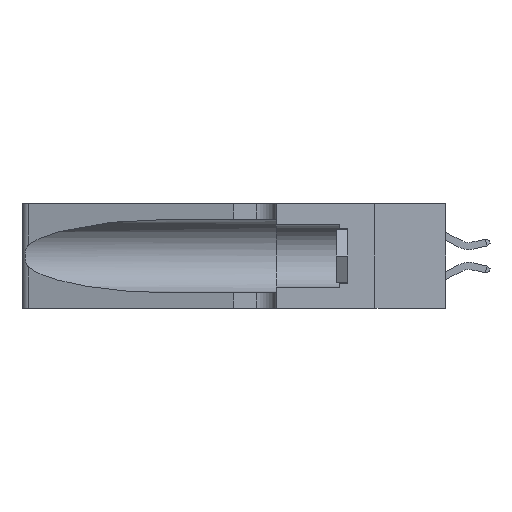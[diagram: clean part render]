
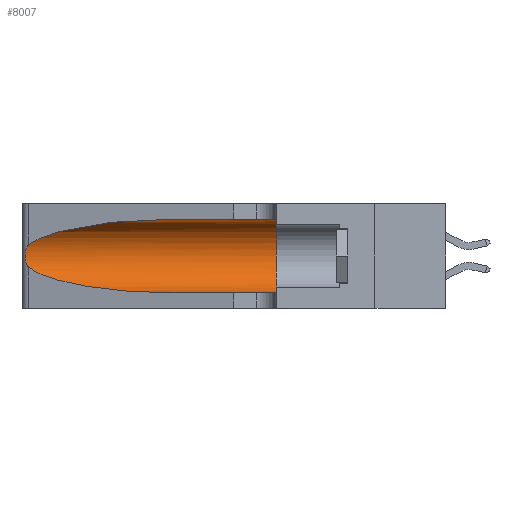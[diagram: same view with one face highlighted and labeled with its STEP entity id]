
A CAD part, left-side view. The second image highlights one B-rep face of the part: STEP entity #8007.
In plain terms, the highlighted cylindrical face has radius 3.308 mm (diameter 6.617 mm), a partial arc.
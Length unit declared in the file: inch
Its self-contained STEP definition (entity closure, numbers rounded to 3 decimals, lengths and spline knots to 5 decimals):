
#169 = VERTEX_POINT ( 'NONE', #20719 ) ;
#1342 = DIRECTION ( 'NONE',  ( 0., -1., 0. ) ) ;
#2211 = CARTESIAN_POINT ( 'NONE',  ( 0.25639, 1.23186, 0.15144 ) ) ;
#2343 = ORIENTED_EDGE ( 'NONE', *, *, #20347, .F. ) ;
#2468 = ORIENTED_EDGE ( 'NONE', *, *, #5573, .T. ) ;
#2977 = CARTESIAN_POINT ( 'NONE',  ( 0.1305, 0.35, 0.185 ) ) ;
#4000 = CARTESIAN_POINT ( 'NONE',  ( 0.1305, 1.61858, 0.31525 ) ) ;
#4860 = CARTESIAN_POINT ( 'NONE',  ( 0.25487, 1.22718, 0.14631 ) ) ;
#5573 = EDGE_CURVE ( 'NONE', #169, #20255, #29001, .T. ) ;
#5644 = CYLINDRICAL_SURFACE ( 'NONE', #11608, 0.13025 ) ;
#5645 = DIRECTION ( 'NONE',  ( 0., 0., 1. ) ) ;
#7001 = CARTESIAN_POINT ( 'NONE',  ( 0.18966, 0.96281, 0.05475 ) ) ;
#7063 = ORIENTED_EDGE ( 'NONE', *, *, #15074, .F. ) ;
#7154 = VERTEX_POINT ( 'NONE', #13464 ) ;
#7499 = CARTESIAN_POINT ( 'NONE',  ( 0.25639, 1.23184, 0.21858 ) ) ;
#7593 = EDGE_LOOP ( 'NONE', ( #31886, #2468, #28564, #13118, #7063, #2343 ) ) ;
#7702 =( BOUNDED_CURVE ( )  B_SPLINE_CURVE ( 3, ( #12294, #23105, #7001, #25785 ),
 .UNSPECIFIED., .F., .T. ) 
 B_SPLINE_CURVE_WITH_KNOTS ( ( 4, 4 ),
 ( 3.44316, 4.71239 ),
 .UNSPECIFIED. ) 
 CURVE ( )  GEOMETRIC_REPRESENTATION_ITEM ( )  RATIONAL_B_SPLINE_CURVE ( ( 1., 0.87, 0.87, 1. ) ) 
 REPRESENTATION_ITEM ( '' )  );
#8007 = ADVANCED_FACE ( 'NONE', ( #19997 ), #5644, .F. ) ;
#8561 = CARTESIAN_POINT ( 'NONE',  ( 0.1305, 1.61858, 0.185 ) ) ;
#8841 = CARTESIAN_POINT ( 'NONE',  ( 0.1305, 0.72297, 0.31525 ) ) ;
#9231 = VECTOR ( 'NONE', #22818, 39.37008 ) ;
#9441 = VECTOR ( 'NONE', #1342, 39.37008 ) ;
#10074 = LINE ( 'NONE', #20116, #9231 ) ;
#10198 = CARTESIAN_POINT ( 'NONE',  ( 0.25854, 1.2359, 0.20912 ) ) ;
#11608 = AXIS2_PLACEMENT_3D ( 'NONE', #8561, #19265, #27364 ) ;
#12294 = CARTESIAN_POINT ( 'NONE',  ( 0.25487, 1.22718, 0.14631 ) ) ;
#12540 = CARTESIAN_POINT ( 'NONE',  ( 0.1305, 0.35, 0.05475 ) ) ;
#12790 = CARTESIAN_POINT ( 'NONE',  ( 0.25555, 1.22994, 0.2215 ) ) ;
#12916 = CARTESIAN_POINT ( 'NONE',  ( 0.26075, 1.23896, 0.19203 ) ) ;
#13118 = ORIENTED_EDGE ( 'NONE', *, *, #30376, .T. ) ;
#13464 = CARTESIAN_POINT ( 'NONE',  ( 0.1305, 0.35, 0.31525 ) ) ;
#15074 = EDGE_CURVE ( 'NONE', #7154, #19864, #25569, .T. ) ;
#15616 = CARTESIAN_POINT ( 'NONE',  ( 0.26017, 1.23833, 0.17102 ) ) ;
#15827 = CARTESIAN_POINT ( 'NONE',  ( 0.18966, 0.96281, 0.31525 ) ) ;
#18191 = CARTESIAN_POINT ( 'NONE',  ( 0.25487, 1.22718, 0.22369 ) ) ;
#18312 = CARTESIAN_POINT ( 'NONE',  ( 0.25789, 1.23486, 0.15765 ) ) ;
#18505 = CARTESIAN_POINT ( 'NONE',  ( 0.25487, 1.22718, 0.22369 ) ) ;
#19265 = DIRECTION ( 'NONE',  ( 0., -1., 0. ) ) ;
#19864 = VERTEX_POINT ( 'NONE', #12540 ) ;
#19997 = FACE_OUTER_BOUND ( 'NONE', #7593, .T. ) ;
#20022 = EDGE_CURVE ( 'NONE', #31368, #169, #32576, .T. ) ;
#20116 = CARTESIAN_POINT ( 'NONE',  ( 0.1305, 1.61858, 0.05475 ) ) ;
#20255 = VERTEX_POINT ( 'NONE', #22509 ) ;
#20347 = EDGE_CURVE ( 'NONE', #31368, #7154, #30832, .T. ) ;
#20719 = CARTESIAN_POINT ( 'NONE',  ( 0.25487, 1.22718, 0.22369 ) ) ;
#21019 = CARTESIAN_POINT ( 'NONE',  ( 0.25555, 1.22993, 0.14849 ) ) ;
#21792 = DIRECTION ( 'NONE',  ( 0., 1., 0. ) ) ;
#22204 = CARTESIAN_POINT ( 'NONE',  ( 0.1305, 0.72297, 0.05475 ) ) ;
#22509 = CARTESIAN_POINT ( 'NONE',  ( 0.25487, 1.22718, 0.14631 ) ) ;
#22818 = DIRECTION ( 'NONE',  ( 0., -1., 0. ) ) ;
#23105 = CARTESIAN_POINT ( 'NONE',  ( 0.2373, 1.15595, 0.08982 ) ) ;
#23669 = VERTEX_POINT ( 'NONE', #22204 ) ;
#25569 = CIRCLE ( 'NONE', #34144, 0.13025 ) ;
#25785 = CARTESIAN_POINT ( 'NONE',  ( 0.1305, 0.72297, 0.05475 ) ) ;
#26296 = CARTESIAN_POINT ( 'NONE',  ( 0.25787, 1.23484, 0.2124 ) ) ;
#26506 = CARTESIAN_POINT ( 'NONE',  ( 0.1305, 0.72297, 0.31525 ) ) ;
#27364 = DIRECTION ( 'NONE',  ( 0., 0., -1. ) ) ;
#28564 = ORIENTED_EDGE ( 'NONE', *, *, #30864, .T. ) ;
#28977 = CARTESIAN_POINT ( 'NONE',  ( 0.26018, 1.23835, 0.19895 ) ) ;
#29001 = B_SPLINE_CURVE_WITH_KNOTS ( 'NONE', 3,
 ( #18191, #12790, #7499, #26296, #10198, #28977, #12916, #31622, #15616, #34282, #18312, #2211, #21019, #4860 ),
 .UNSPECIFIED., .F., .F.,
 ( 4, 2, 2, 2, 2, 2, 4 ),
 ( 0., 0.00027, 0.00053, 0.00107, 0.0016, 0.00187, 0.00214 ),
 .UNSPECIFIED. ) ;
#30376 = EDGE_CURVE ( 'NONE', #23669, #19864, #10074, .T. ) ;
#30832 = LINE ( 'NONE', #4000, #9441 ) ;
#30864 = EDGE_CURVE ( 'NONE', #20255, #23669, #7702, .T. ) ;
#31368 = VERTEX_POINT ( 'NONE', #8841 ) ;
#31622 = CARTESIAN_POINT ( 'NONE',  ( 0.26075, 1.23896, 0.178 ) ) ;
#31886 = ORIENTED_EDGE ( 'NONE', *, *, #20022, .T. ) ;
#32576 =( BOUNDED_CURVE ( )  B_SPLINE_CURVE ( 3, ( #26506, #15827, #34495, #18505 ),
 .UNSPECIFIED., .F., .F. ) 
 B_SPLINE_CURVE_WITH_KNOTS ( ( 4, 4 ),
 ( 1.5708, 2.84003 ),
 .UNSPECIFIED. ) 
 CURVE ( )  GEOMETRIC_REPRESENTATION_ITEM ( )  RATIONAL_B_SPLINE_CURVE ( ( 1., 0.87, 0.87, 1. ) ) 
 REPRESENTATION_ITEM ( '' )  );
#34144 = AXIS2_PLACEMENT_3D ( 'NONE', #2977, #21792, #5645 ) ;
#34282 = CARTESIAN_POINT ( 'NONE',  ( 0.25856, 1.23593, 0.16098 ) ) ;
#34495 = CARTESIAN_POINT ( 'NONE',  ( 0.2373, 1.15595, 0.28018 ) ) ;
